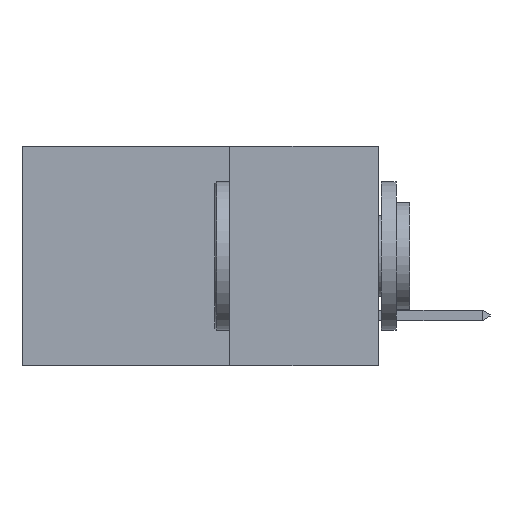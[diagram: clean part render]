
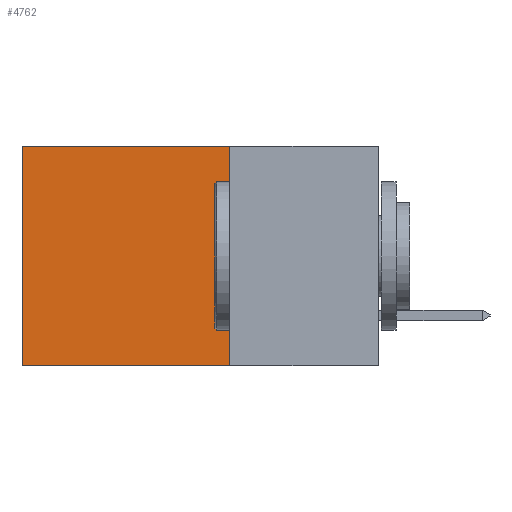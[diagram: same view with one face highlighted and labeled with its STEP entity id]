
A CAD part, left-side view. The second image highlights one B-rep face of the part: STEP entity #4762.
In plain terms, the highlighted planar face has unit normal (-1, 0, 0).
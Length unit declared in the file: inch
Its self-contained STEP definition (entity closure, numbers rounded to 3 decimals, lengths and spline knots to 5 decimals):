
#12 = EDGE_LOOP ( 'NONE', ( #5826, #587, #10973, #6312 ) ) ;
#287 = EDGE_CURVE ( 'NONE', #9288, #323, #11363, .T. ) ;
#323 = VERTEX_POINT ( 'NONE', #2128 ) ;
#587 = ORIENTED_EDGE ( 'NONE', *, *, #287, .F. ) ;
#768 = EDGE_CURVE ( 'NONE', #2326, #9288, #3264, .T. ) ;
#1041 = DIRECTION ( 'NONE',  ( 0., 1., 0. ) ) ;
#1197 = CARTESIAN_POINT ( 'NONE',  ( 0.2615, 0.25, -0.37 ) ) ;
#1235 = VECTOR ( 'NONE', #11515, 39.37008 ) ;
#1487 = CARTESIAN_POINT ( 'NONE',  ( 0.2615, 0.6, 0. ) ) ;
#2128 = CARTESIAN_POINT ( 'NONE',  ( 0.2615, 0.6, -0.37 ) ) ;
#2326 = VERTEX_POINT ( 'NONE', #15669 ) ;
#3264 = LINE ( 'NONE', #8573, #17857 ) ;
#4762 = ADVANCED_FACE ( 'NONE', ( #16253 ), #8775, .F. ) ;
#5062 = VECTOR ( 'NONE', #1041, 39.37008 ) ;
#5826 = ORIENTED_EDGE ( 'NONE', *, *, #15428, .T. ) ;
#6312 = ORIENTED_EDGE ( 'NONE', *, *, #11364, .T. ) ;
#7167 = CARTESIAN_POINT ( 'NONE',  ( 0.2615, 0.6, -0.37 ) ) ;
#8313 = DIRECTION ( 'NONE',  ( 0., 0., -1. ) ) ;
#8444 = DIRECTION ( 'NONE',  ( 0., 0., -1. ) ) ;
#8497 = DIRECTION ( 'NONE',  ( 1., 0., 0. ) ) ;
#8517 = CARTESIAN_POINT ( 'NONE',  ( 0.2615, 0.25, -0.37 ) ) ;
#8573 = CARTESIAN_POINT ( 'NONE',  ( 0.2615, 0.25, -0.37 ) ) ;
#8775 = PLANE ( 'NONE',  #15013 ) ;
#9288 = VERTEX_POINT ( 'NONE', #15683 ) ;
#9408 = DIRECTION ( 'NONE',  ( 0., 1., 0. ) ) ;
#10312 = VECTOR ( 'NONE', #9408, 39.37008 ) ;
#10948 = LINE ( 'NONE', #7167, #1235 ) ;
#10973 = ORIENTED_EDGE ( 'NONE', *, *, #768, .F. ) ;
#11363 = LINE ( 'NONE', #1197, #5062 ) ;
#11364 = EDGE_CURVE ( 'NONE', #2326, #12271, #17305, .T. ) ;
#11515 = DIRECTION ( 'NONE',  ( 0., 0., -1. ) ) ;
#12271 = VERTEX_POINT ( 'NONE', #1487 ) ;
#15013 = AXIS2_PLACEMENT_3D ( 'NONE', #8517, #8497, #8444 ) ;
#15428 = EDGE_CURVE ( 'NONE', #12271, #323, #10948, .T. ) ;
#15669 = CARTESIAN_POINT ( 'NONE',  ( 0.2615, 0.25, 0. ) ) ;
#15683 = CARTESIAN_POINT ( 'NONE',  ( 0.2615, 0.25, -0.37 ) ) ;
#16253 = FACE_OUTER_BOUND ( 'NONE', #12, .T. ) ;
#17305 = LINE ( 'NONE', #17828, #10312 ) ;
#17828 = CARTESIAN_POINT ( 'NONE',  ( 0.2615, 0.25, 0. ) ) ;
#17857 = VECTOR ( 'NONE', #8313, 39.37008 ) ;
